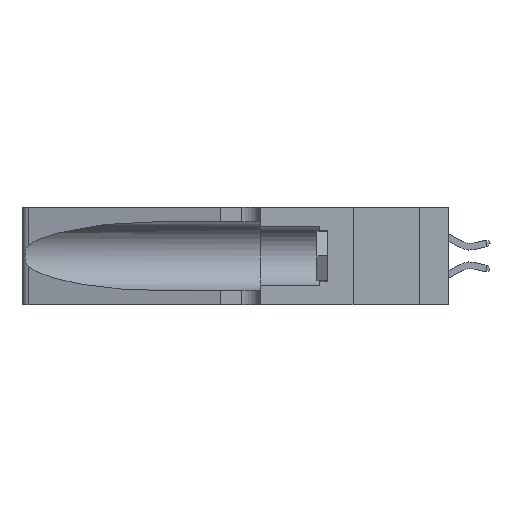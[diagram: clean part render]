
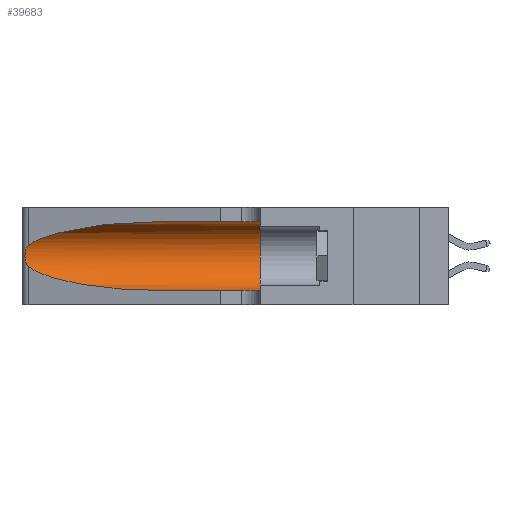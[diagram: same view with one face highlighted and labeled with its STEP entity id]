
A CAD part, left-side view. The second image highlights one B-rep face of the part: STEP entity #39683.
In plain terms, the highlighted cylindrical face has radius 3.308 mm (diameter 6.617 mm), a partial arc.
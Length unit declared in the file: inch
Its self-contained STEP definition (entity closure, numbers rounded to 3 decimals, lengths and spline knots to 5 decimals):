
#102 = CARTESIAN_POINT ( 'NONE',  ( 0.26075, 1.23896, 0.19203 ) ) ;
#2891 = CARTESIAN_POINT ( 'NONE',  ( 0.25555, 1.22994, 0.2215 ) ) ;
#2905 = CARTESIAN_POINT ( 'NONE',  ( 0.25487, 1.22718, 0.14631 ) ) ;
#2975 = VERTEX_POINT ( 'NONE', #32345 ) ;
#3024 = EDGE_LOOP ( 'NONE', ( #6477, #38118, #21078, #4182, #6946, #21106 ) ) ;
#3425 = CARTESIAN_POINT ( 'NONE',  ( 0.26075, 1.23896, 0.178 ) ) ;
#3739 = VERTEX_POINT ( 'NONE', #6286 ) ;
#4182 = ORIENTED_EDGE ( 'NONE', *, *, #12990, .T. ) ;
#5697 = DIRECTION ( 'NONE',  ( 0., -1., 0. ) ) ;
#6065 = CARTESIAN_POINT ( 'NONE',  ( 0.25856, 1.23593, 0.16098 ) ) ;
#6212 = CARTESIAN_POINT ( 'NONE',  ( 0.1305, 0.35, 0.31525 ) ) ;
#6286 = CARTESIAN_POINT ( 'NONE',  ( 0.1305, 0.72297, 0.05475 ) ) ;
#6325 = CARTESIAN_POINT ( 'NONE',  ( 0.26018, 1.23835, 0.19895 ) ) ;
#6383 = EDGE_CURVE ( 'NONE', #31674, #2975, #27658, .T. ) ;
#6477 = ORIENTED_EDGE ( 'NONE', *, *, #6383, .T. ) ;
#6696 = DIRECTION ( 'NONE',  ( 0., 0., 1. ) ) ;
#6946 = ORIENTED_EDGE ( 'NONE', *, *, #21517, .F. ) ;
#7524 = CARTESIAN_POINT ( 'NONE',  ( 0.18966, 0.96281, 0.05475 ) ) ;
#7641 = DIRECTION ( 'NONE',  ( 0., -1., 0. ) ) ;
#7953 = CARTESIAN_POINT ( 'NONE',  ( 0.2373, 1.15595, 0.08982 ) ) ;
#8248 = AXIS2_PLACEMENT_3D ( 'NONE', #26844, #7641, #10860 ) ;
#8325 = CARTESIAN_POINT ( 'NONE',  ( 0.2373, 1.15595, 0.28018 ) ) ;
#8648 = CARTESIAN_POINT ( 'NONE',  ( 0.25487, 1.22718, 0.14631 ) ) ;
#9411 = CARTESIAN_POINT ( 'NONE',  ( 0.25639, 1.23184, 0.21858 ) ) ;
#9653 = B_SPLINE_CURVE_WITH_KNOTS ( 'NONE', 3,
 ( #38081, #2891, #9411, #35428, #41279, #6325, #102, #3425, #18941, #6065, #22180, #25649, #32110, #12887 ),
 .UNSPECIFIED., .F., .F.,
 ( 4, 2, 2, 2, 2, 2, 4 ),
 ( 0., 0.00027, 0.00053, 0.00107, 0.0016, 0.00187, 0.00214 ),
 .UNSPECIFIED. ) ;
#10023 = CARTESIAN_POINT ( 'NONE',  ( 0.1305, 1.61858, 0.31525 ) ) ;
#10145 =( BOUNDED_CURVE ( )  B_SPLINE_CURVE ( 3, ( #2905, #7953, #7524, #14117 ),
 .UNSPECIFIED., .F., .F. ) 
 B_SPLINE_CURVE_WITH_KNOTS ( ( 4, 4 ),
 ( 3.44316, 4.71239 ),
 .UNSPECIFIED. ) 
 CURVE ( )  GEOMETRIC_REPRESENTATION_ITEM ( )  RATIONAL_B_SPLINE_CURVE ( ( 1., 0.87, 0.87, 1. ) ) 
 REPRESENTATION_ITEM ( '' )  );
#10345 = FACE_OUTER_BOUND ( 'NONE', #3024, .T. ) ;
#10515 = CARTESIAN_POINT ( 'NONE',  ( 0.1305, 0.72297, 0.31525 ) ) ;
#10860 = DIRECTION ( 'NONE',  ( 0., 0., -1. ) ) ;
#10985 = LINE ( 'NONE', #10023, #28072 ) ;
#11635 = VECTOR ( 'NONE', #5697, 39.37008 ) ;
#12069 = CARTESIAN_POINT ( 'NONE',  ( 0.1305, 0.35, 0.185 ) ) ;
#12631 = LINE ( 'NONE', #21812, #11635 ) ;
#12887 = CARTESIAN_POINT ( 'NONE',  ( 0.25487, 1.22718, 0.14631 ) ) ;
#12990 = EDGE_CURVE ( 'NONE', #3739, #39580, #12631, .T. ) ;
#14117 = CARTESIAN_POINT ( 'NONE',  ( 0.1305, 0.72297, 0.05475 ) ) ;
#14915 = EDGE_CURVE ( 'NONE', #18265, #3739, #10145, .T. ) ;
#18265 = VERTEX_POINT ( 'NONE', #8648 ) ;
#18725 = EDGE_CURVE ( 'NONE', #31674, #23894, #10985, .T. ) ;
#18941 = CARTESIAN_POINT ( 'NONE',  ( 0.26017, 1.23833, 0.17102 ) ) ;
#19278 = CARTESIAN_POINT ( 'NONE',  ( 0.1305, 0.35, 0.05475 ) ) ;
#21078 = ORIENTED_EDGE ( 'NONE', *, *, #14915, .T. ) ;
#21106 = ORIENTED_EDGE ( 'NONE', *, *, #18725, .F. ) ;
#21239 = CARTESIAN_POINT ( 'NONE',  ( 0.1305, 0.72297, 0.31525 ) ) ;
#21517 = EDGE_CURVE ( 'NONE', #23894, #39580, #32867, .T. ) ;
#21812 = CARTESIAN_POINT ( 'NONE',  ( 0.1305, 1.61858, 0.05475 ) ) ;
#22180 = CARTESIAN_POINT ( 'NONE',  ( 0.25789, 1.23486, 0.15765 ) ) ;
#23894 = VERTEX_POINT ( 'NONE', #6212 ) ;
#25649 = CARTESIAN_POINT ( 'NONE',  ( 0.25639, 1.23186, 0.15144 ) ) ;
#26844 = CARTESIAN_POINT ( 'NONE',  ( 0.1305, 1.61858, 0.185 ) ) ;
#27658 =( BOUNDED_CURVE ( )  B_SPLINE_CURVE ( 3, ( #21239, #37149, #8325, #33983 ),
 .UNSPECIFIED., .F., .F. ) 
 B_SPLINE_CURVE_WITH_KNOTS ( ( 4, 4 ),
 ( 1.5708, 2.84003 ),
 .UNSPECIFIED. ) 
 CURVE ( )  GEOMETRIC_REPRESENTATION_ITEM ( )  RATIONAL_B_SPLINE_CURVE ( ( 1., 0.87, 0.87, 1. ) ) 
 REPRESENTATION_ITEM ( '' )  );
#28072 = VECTOR ( 'NONE', #38954, 39.37008 ) ;
#28549 = AXIS2_PLACEMENT_3D ( 'NONE', #12069, #37929, #6696 ) ;
#31461 = CYLINDRICAL_SURFACE ( 'NONE', #8248, 0.13025 ) ;
#31516 = EDGE_CURVE ( 'NONE', #2975, #18265, #9653, .T. ) ;
#31674 = VERTEX_POINT ( 'NONE', #10515 ) ;
#32110 = CARTESIAN_POINT ( 'NONE',  ( 0.25555, 1.22993, 0.14849 ) ) ;
#32345 = CARTESIAN_POINT ( 'NONE',  ( 0.25487, 1.22718, 0.22369 ) ) ;
#32867 = CIRCLE ( 'NONE', #28549, 0.13025 ) ;
#33983 = CARTESIAN_POINT ( 'NONE',  ( 0.25487, 1.22718, 0.22369 ) ) ;
#35428 = CARTESIAN_POINT ( 'NONE',  ( 0.25787, 1.23484, 0.2124 ) ) ;
#37149 = CARTESIAN_POINT ( 'NONE',  ( 0.18966, 0.96281, 0.31525 ) ) ;
#37929 = DIRECTION ( 'NONE',  ( 0., 1., 0. ) ) ;
#38081 = CARTESIAN_POINT ( 'NONE',  ( 0.25487, 1.22718, 0.22369 ) ) ;
#38118 = ORIENTED_EDGE ( 'NONE', *, *, #31516, .T. ) ;
#38954 = DIRECTION ( 'NONE',  ( 0., -1., 0. ) ) ;
#39580 = VERTEX_POINT ( 'NONE', #19278 ) ;
#39683 = ADVANCED_FACE ( 'NONE', ( #10345 ), #31461, .F. ) ;
#41279 = CARTESIAN_POINT ( 'NONE',  ( 0.25854, 1.2359, 0.20912 ) ) ;
